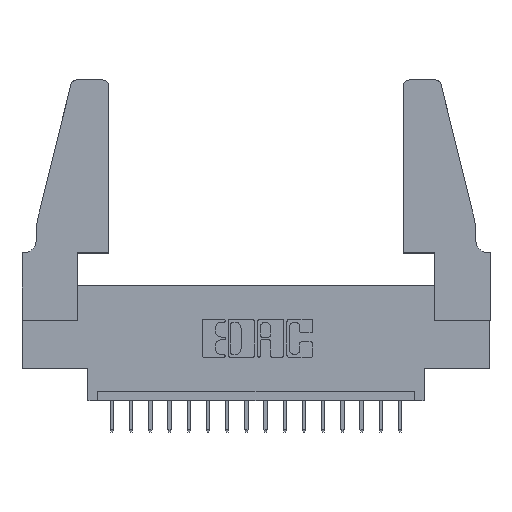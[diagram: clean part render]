
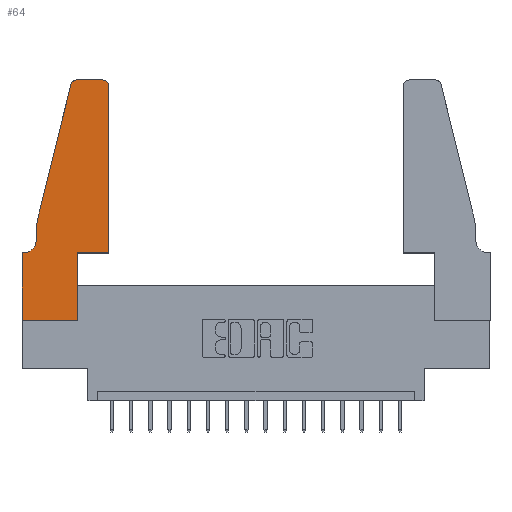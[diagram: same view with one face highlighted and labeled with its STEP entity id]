
A CAD part, top view. The second image highlights one B-rep face of the part: STEP entity #64.
In plain terms, the highlighted planar face has unit normal (0, 0, 1).
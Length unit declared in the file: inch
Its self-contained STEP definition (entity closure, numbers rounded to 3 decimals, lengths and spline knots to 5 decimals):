
#64 = ADVANCED_FACE ( 'NONE', ( #13028 ), #1666, .T. ) ;
#120 = EDGE_CURVE ( 'NONE', #16287, #1702, #3301, .T. ) ;
#231 = VERTEX_POINT ( 'NONE', #8094 ) ;
#631 = VECTOR ( 'NONE', #6179, 39.37008 ) ;
#711 = CARTESIAN_POINT ( 'NONE',  ( 0.4505, 1.22, 0.37 ) ) ;
#803 = CARTESIAN_POINT ( 'NONE',  ( 0.284, 1.25, 0.37 ) ) ;
#809 = CARTESIAN_POINT ( 'NONE',  ( 0.284, 1.22, 0.37 ) ) ;
#1006 = LINE ( 'NONE', #2364, #6182 ) ;
#1252 = EDGE_CURVE ( 'NONE', #7284, #12504, #4580, .T. ) ;
#1374 = CARTESIAN_POINT ( 'NONE',  ( 0.4205, 1.25, 0.37 ) ) ;
#1416 = CARTESIAN_POINT ( 'NONE',  ( 0.4505, 0.35, 0.37 ) ) ;
#1519 = VERTEX_POINT ( 'NONE', #1374 ) ;
#1579 = DIRECTION ( 'NONE',  ( -1., 0., 0. ) ) ;
#1666 = PLANE ( 'NONE',  #8746 ) ;
#1702 = VERTEX_POINT ( 'NONE', #16991 ) ;
#2016 = ORIENTED_EDGE ( 'NONE', *, *, #3457, .T. ) ;
#2023 = LINE ( 'NONE', #4997, #17600 ) ;
#2139 = DIRECTION ( 'NONE',  ( 0., 0., 1. ) ) ;
#2148 = CARTESIAN_POINT ( 'NONE',  ( 0.0055, 0.35, 0.37 ) ) ;
#2316 = VECTOR ( 'NONE', #1579, 39.37008 ) ;
#2364 = CARTESIAN_POINT ( 'NONE',  ( 0.0755, 0.35, 0.37 ) ) ;
#2432 = EDGE_CURVE ( 'NONE', #1702, #7284, #13813, .T. ) ;
#2462 = VECTOR ( 'NONE', #17158, 39.37008 ) ;
#2811 = ORIENTED_EDGE ( 'NONE', *, *, #14723, .T. ) ;
#3022 = ORIENTED_EDGE ( 'NONE', *, *, #13734, .T. ) ;
#3301 = LINE ( 'NONE', #15640, #14975 ) ;
#3360 = DIRECTION ( 'NONE',  ( 1., 0., 0. ) ) ;
#3384 = DIRECTION ( 'NONE',  ( 0., 0., -1. ) ) ;
#3457 = EDGE_CURVE ( 'NONE', #13038, #16545, #17210, .T. ) ;
#3572 = CARTESIAN_POINT ( 'NONE',  ( 0.4205, 1.22, 0.37 ) ) ;
#3590 = DIRECTION ( 'NONE',  ( 1., 0., 0. ) ) ;
#3663 = VECTOR ( 'NONE', #5067, 39.37008 ) ;
#4146 = ORIENTED_EDGE ( 'NONE', *, *, #2432, .T. ) ;
#4253 = VECTOR ( 'NONE', #9406, 39.37008 ) ;
#4333 = EDGE_CURVE ( 'NONE', #13137, #16287, #2023, .T. ) ;
#4479 = LINE ( 'NONE', #17920, #4253 ) ;
#4580 = LINE ( 'NONE', #1416, #11287 ) ;
#4631 = CIRCLE ( 'NONE', #7931, 0.07 ) ;
#4729 = LINE ( 'NONE', #5928, #3663 ) ;
#4734 = CIRCLE ( 'NONE', #11352, 0.03 ) ;
#4830 = LINE ( 'NONE', #11460, #2462 ) ;
#4997 = CARTESIAN_POINT ( 'NONE',  ( 0., 0., 0.37 ) ) ;
#5000 = VERTEX_POINT ( 'NONE', #9007 ) ;
#5067 = DIRECTION ( 'NONE',  ( 0., 1., 0. ) ) ;
#5231 = ORIENTED_EDGE ( 'NONE', *, *, #15152, .T. ) ;
#5237 = CARTESIAN_POINT ( 'NONE',  ( 0.2865, 0.35, 0.37 ) ) ;
#5379 = DIRECTION ( 'NONE',  ( 1., 0., 0. ) ) ;
#5598 = CARTESIAN_POINT ( 'NONE',  ( 0.25487, 1.22718, 0.37 ) ) ;
#5721 = CARTESIAN_POINT ( 'NONE',  ( 0.2605, 1.25, 0.37 ) ) ;
#5768 = CARTESIAN_POINT ( 'NONE',  ( 0.4505, 0.35, 0.37 ) ) ;
#5928 = CARTESIAN_POINT ( 'NONE',  ( 0.4505, 0.35, 0.37 ) ) ;
#6179 = DIRECTION ( 'NONE',  ( 0., 1., 0. ) ) ;
#6182 = VECTOR ( 'NONE', #9435, 39.37008 ) ;
#6298 = DIRECTION ( 'NONE',  ( 0., 0., 1. ) ) ;
#6476 = CARTESIAN_POINT ( 'NONE',  ( 0., 0., 0.37 ) ) ;
#6911 = EDGE_CURVE ( 'NONE', #12504, #16943, #4729, .T. ) ;
#7284 = VERTEX_POINT ( 'NONE', #5237 ) ;
#7312 = DIRECTION ( 'NONE',  ( 1., 0., 0. ) ) ;
#7537 = DIRECTION ( 'NONE',  ( 0., 0., 1. ) ) ;
#7931 = AXIS2_PLACEMENT_3D ( 'NONE', #16092, #3384, #17227 ) ;
#8094 = CARTESIAN_POINT ( 'NONE',  ( 0.0755, 0.42, 0.37 ) ) ;
#8199 = EDGE_CURVE ( 'NONE', #16545, #5000, #4479, .T. ) ;
#8746 = AXIS2_PLACEMENT_3D ( 'NONE', #15529, #2139, #3590 ) ;
#8855 = CARTESIAN_POINT ( 'NONE',  ( 0.2865, 0.35, 0.37 ) ) ;
#9007 = CARTESIAN_POINT ( 'NONE',  ( 0.0755, 0.5, 0.37 ) ) ;
#9406 = DIRECTION ( 'NONE',  ( -0.239, -0.971, 0. ) ) ;
#9435 = DIRECTION ( 'NONE',  ( -1., 0., 0. ) ) ;
#9802 = ORIENTED_EDGE ( 'NONE', *, *, #120, .T. ) ;
#10515 = DIRECTION ( 'NONE',  ( 1., 0., 0. ) ) ;
#10904 = EDGE_CURVE ( 'NONE', #231, #17765, #4631, .T. ) ;
#11287 = VECTOR ( 'NONE', #5379, 39.37008 ) ;
#11352 = AXIS2_PLACEMENT_3D ( 'NONE', #3572, #7537, #10515 ) ;
#11408 = LINE ( 'NONE', #5721, #2316 ) ;
#11460 = CARTESIAN_POINT ( 'NONE',  ( 0.0755, 0.5, 0.37 ) ) ;
#11581 = ORIENTED_EDGE ( 'NONE', *, *, #8199, .T. ) ;
#11959 = CARTESIAN_POINT ( 'NONE',  ( 0., 0.35, 0.37 ) ) ;
#12142 = AXIS2_PLACEMENT_3D ( 'NONE', #809, #6298, #3360 ) ;
#12312 = ORIENTED_EDGE ( 'NONE', *, *, #6911, .T. ) ;
#12504 = VERTEX_POINT ( 'NONE', #5768 ) ;
#13028 = FACE_OUTER_BOUND ( 'NONE', #17694, .T. ) ;
#13038 = VERTEX_POINT ( 'NONE', #803 ) ;
#13102 = DIRECTION ( 'NONE',  ( 0., -1., 0. ) ) ;
#13137 = VERTEX_POINT ( 'NONE', #11959 ) ;
#13426 = ORIENTED_EDGE ( 'NONE', *, *, #10904, .T. ) ;
#13734 = EDGE_CURVE ( 'NONE', #16943, #1519, #4734, .T. ) ;
#13813 = LINE ( 'NONE', #8855, #631 ) ;
#14723 = EDGE_CURVE ( 'NONE', #1519, #13038, #11408, .T. ) ;
#14975 = VECTOR ( 'NONE', #7312, 39.37008 ) ;
#15152 = EDGE_CURVE ( 'NONE', #17765, #13137, #1006, .T. ) ;
#15199 = ORIENTED_EDGE ( 'NONE', *, *, #1252, .T. ) ;
#15529 = CARTESIAN_POINT ( 'NONE',  ( 0., 0.35, 0.37 ) ) ;
#15640 = CARTESIAN_POINT ( 'NONE',  ( 0., 0., 0.37 ) ) ;
#16092 = CARTESIAN_POINT ( 'NONE',  ( 0.0055, 0.42, 0.37 ) ) ;
#16287 = VERTEX_POINT ( 'NONE', #6476 ) ;
#16545 = VERTEX_POINT ( 'NONE', #5598 ) ;
#16943 = VERTEX_POINT ( 'NONE', #711 ) ;
#16991 = CARTESIAN_POINT ( 'NONE',  ( 0.2865, 0., 0.37 ) ) ;
#17158 = DIRECTION ( 'NONE',  ( 0., -1., 0. ) ) ;
#17210 = CIRCLE ( 'NONE', #12142, 0.03 ) ;
#17227 = DIRECTION ( 'NONE',  ( -1., 0., 0. ) ) ;
#17437 = ORIENTED_EDGE ( 'NONE', *, *, #17616, .T. ) ;
#17600 = VECTOR ( 'NONE', #13102, 39.37008 ) ;
#17616 = EDGE_CURVE ( 'NONE', #5000, #231, #4830, .T. ) ;
#17668 = ORIENTED_EDGE ( 'NONE', *, *, #4333, .T. ) ;
#17694 = EDGE_LOOP ( 'NONE', ( #2811, #2016, #11581, #17437, #13426, #5231, #17668, #9802, #4146, #15199, #12312, #3022 ) ) ;
#17765 = VERTEX_POINT ( 'NONE', #2148 ) ;
#17920 = CARTESIAN_POINT ( 'NONE',  ( 0.0755, 0.5, 0.37 ) ) ;
